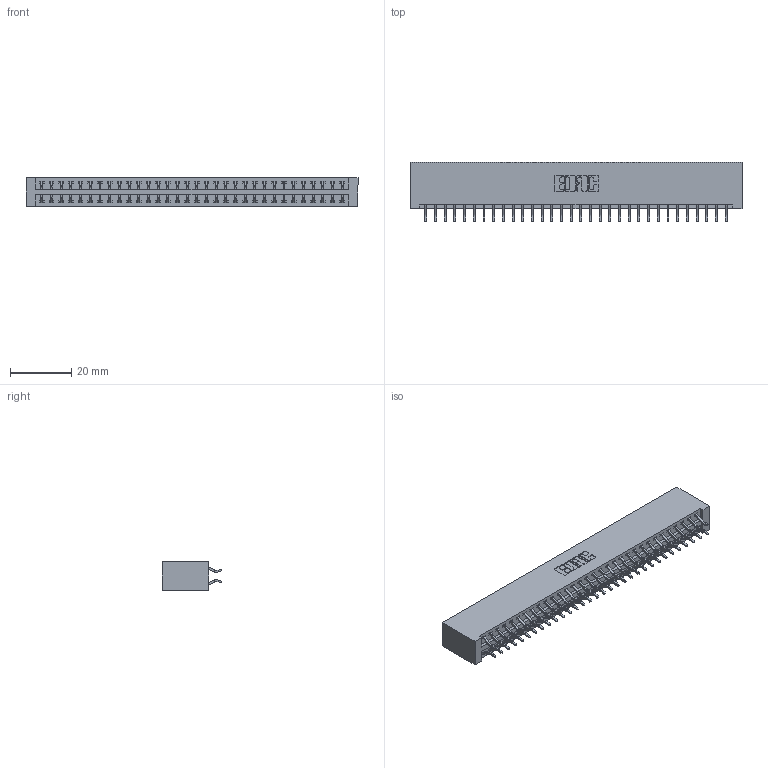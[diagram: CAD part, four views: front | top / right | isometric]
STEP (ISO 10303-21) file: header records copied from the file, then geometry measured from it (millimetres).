
FILE_DESCRIPTION (( 'STEP AP203' ), '1' );
FILE_NAME ('346-064-556-201.STEP', '2022-05-24T15:50:30', ( '' ), ( '' ), 'SwSTEP 2.0', 'SolidWorks 2020', '' );
FILE_SCHEMA (( 'CONFIG_CONTROL_DESIGN' ));
Length unit declared in the file: inch
Products named in the file (3): 345-292-001_556 Tail; 346-064-556-201; 346 Part_No Mounting Lugs
Assembly tree (65 placements, depth 2):
  346-064-556-201
    346 Part_No Mounting Lugs
    345-292-001_556 Tail  x64
Bounding box: 108.84 x 19.57 x 9.4 mm (x, y, z)
Volume: 11106.2 mm3; surface area: 15212.8 mm2
Topology: 65 solids, 65 shells, 3826 faces, 11377 edges, 7498 vertices
Faces by surface type: plane 2568, cylinder 1258
Entity records: 22173 total; most frequent: CARTESIAN_POINT 3680, ORIENTED_EDGE 3602, DIRECTION 3277, EDGE_CURVE 1801, VECTOR 1541, LINE 1541, VERTEX_POINT 1198, AXIS2_PLACEMENT_3D 868
